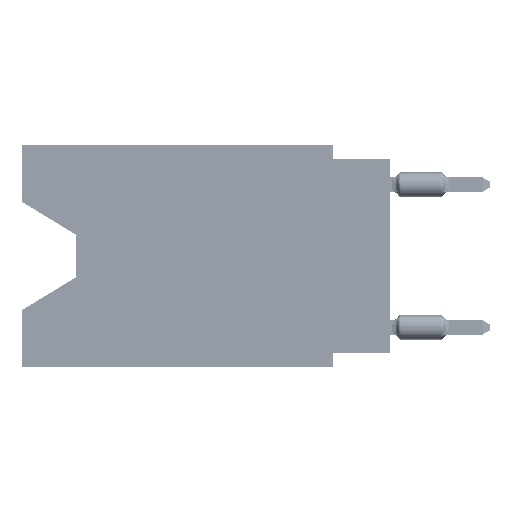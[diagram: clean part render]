
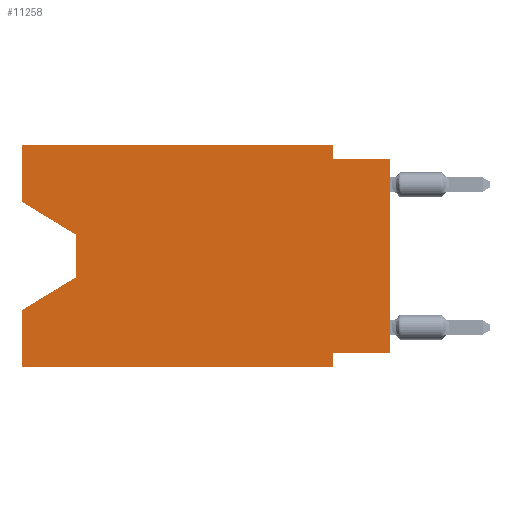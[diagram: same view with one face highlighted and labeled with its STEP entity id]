
A CAD part, left-side view. The second image highlights one B-rep face of the part: STEP entity #11258.
In plain terms, the highlighted planar face has unit normal (-1, 0, 0).
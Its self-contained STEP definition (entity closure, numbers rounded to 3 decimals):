
#1459 = EDGE_CURVE ( 'NONE', #8848, #53704, #19387, .T. ) ;
#1795 = CARTESIAN_POINT ( 'NONE',  ( 0., 2.54, 0. ) ) ;
#1817 = VECTOR ( 'NONE', #56384, 1000. ) ;
#1835 = VERTEX_POINT ( 'NONE', #5808 ) ;
#2385 = EDGE_CURVE ( 'NONE', #43833, #4414, #7277, .T. ) ;
#2601 = CARTESIAN_POINT ( 'NONE',  ( 0., 13.97, -5.893 ) ) ;
#3404 = FACE_OUTER_BOUND ( 'NONE', #23975, .T. ) ;
#3850 = LINE ( 'NONE', #23062, #57773 ) ;
#4297 = CARTESIAN_POINT ( 'NONE',  ( 0., 16.383, -9.906 ) ) ;
#4414 = VERTEX_POINT ( 'NONE', #1795 ) ;
#4616 = DIRECTION ( 'NONE',  ( 0., 1., 0. ) ) ;
#5125 = CARTESIAN_POINT ( 'NONE',  ( 0., 2.54, -9.906 ) ) ;
#5251 = DIRECTION ( 'NONE',  ( 0., -1., 0. ) ) ;
#5705 = CARTESIAN_POINT ( 'NONE',  ( 0., 16.383, -9.906 ) ) ;
#5808 = CARTESIAN_POINT ( 'NONE',  ( 0., 0., -0.635 ) ) ;
#5877 = CARTESIAN_POINT ( 'NONE',  ( 0., 16.383, 0. ) ) ;
#6912 = VERTEX_POINT ( 'NONE', #57296 ) ;
#7214 = DIRECTION ( 'NONE',  ( 0., 0., -1. ) ) ;
#7277 = LINE ( 'NONE', #31486, #11362 ) ;
#8170 = ORIENTED_EDGE ( 'NONE', *, *, #18318, .T. ) ;
#8647 = EDGE_CURVE ( 'NONE', #4414, #37309, #61099, .T. ) ;
#8848 = VERTEX_POINT ( 'NONE', #5705 ) ;
#9595 = ORIENTED_EDGE ( 'NONE', *, *, #14722, .F. ) ;
#11202 = VERTEX_POINT ( 'NONE', #56272 ) ;
#11258 = ADVANCED_FACE ( 'NONE', ( #3404 ), #16633, .F. ) ;
#11362 = VECTOR ( 'NONE', #49459, 1000. ) ;
#11464 = VECTOR ( 'NONE', #43907, 1000. ) ;
#12259 = CARTESIAN_POINT ( 'NONE',  ( 0., 0., -9.271 ) ) ;
#13710 = DIRECTION ( 'NONE',  ( 0., 0., 1. ) ) ;
#14200 = ORIENTED_EDGE ( 'NONE', *, *, #18834, .T. ) ;
#14722 = EDGE_CURVE ( 'NONE', #30793, #43833, #3850, .T. ) ;
#14852 = LINE ( 'NONE', #5125, #23028 ) ;
#14898 = ORIENTED_EDGE ( 'NONE', *, *, #27889, .T. ) ;
#15751 = CARTESIAN_POINT ( 'NONE',  ( 0., 16.383, 0. ) ) ;
#16633 = PLANE ( 'NONE',  #61138 ) ;
#18259 = VECTOR ( 'NONE', #29150, 1000. ) ;
#18318 = EDGE_CURVE ( 'NONE', #54765, #53704, #20858, .T. ) ;
#18834 = EDGE_CURVE ( 'NONE', #30793, #44508, #41213, .T. ) ;
#18895 = EDGE_CURVE ( 'NONE', #11202, #26272, #23185, .T. ) ;
#19387 = LINE ( 'NONE', #5877, #18259 ) ;
#19645 = ORIENTED_EDGE ( 'NONE', *, *, #20628, .T. ) ;
#19694 = VECTOR ( 'NONE', #59568, 1000. ) ;
#20628 = EDGE_CURVE ( 'NONE', #8848, #6912, #62211, .T. ) ;
#20858 = LINE ( 'NONE', #2601, #19694 ) ;
#22007 = ORIENTED_EDGE ( 'NONE', *, *, #57055, .F. ) ;
#22021 = DIRECTION ( 'NONE',  ( 0., -0.855, -0.519 ) ) ;
#23028 = VECTOR ( 'NONE', #48539, 1000. ) ;
#23062 = CARTESIAN_POINT ( 'NONE',  ( 0., 16.383, 0. ) ) ;
#23175 = LINE ( 'NONE', #27587, #49689 ) ;
#23185 = LINE ( 'NONE', #12259, #54922 ) ;
#23975 = EDGE_LOOP ( 'NONE', ( #14200, #14898, #8170, #43128, #19645, #51149, #30018, #38685, #22007, #46009, #32661, #9595 ) ) ;
#25698 = DIRECTION ( 'NONE',  ( 0., 0., 1. ) ) ;
#26272 = VERTEX_POINT ( 'NONE', #46825 ) ;
#27587 = CARTESIAN_POINT ( 'NONE',  ( 0., 0., 0. ) ) ;
#27889 = EDGE_CURVE ( 'NONE', #44508, #54765, #58396, .T. ) ;
#29150 = DIRECTION ( 'NONE',  ( 0., 0., 1. ) ) ;
#29646 = CARTESIAN_POINT ( 'NONE',  ( 0., 16.383, -2.546 ) ) ;
#30018 = ORIENTED_EDGE ( 'NONE', *, *, #18895, .F. ) ;
#30793 = VERTEX_POINT ( 'NONE', #29646 ) ;
#31441 = CARTESIAN_POINT ( 'NONE',  ( 0., 13.97, -5.893 ) ) ;
#31486 = CARTESIAN_POINT ( 'NONE',  ( 0., 16.383, 0. ) ) ;
#32661 = ORIENTED_EDGE ( 'NONE', *, *, #2385, .F. ) ;
#34424 = EDGE_CURVE ( 'NONE', #26272, #6912, #14852, .T. ) ;
#34960 = CARTESIAN_POINT ( 'NONE',  ( 0., 2.54, -0.635 ) ) ;
#34983 = VECTOR ( 'NONE', #5251, 1000. ) ;
#36754 = CARTESIAN_POINT ( 'NONE',  ( 0., 0., -0.635 ) ) ;
#37309 = VERTEX_POINT ( 'NONE', #34960 ) ;
#37951 = CARTESIAN_POINT ( 'NONE',  ( 0., 16.383, -2.546 ) ) ;
#38685 = ORIENTED_EDGE ( 'NONE', *, *, #56535, .T. ) ;
#39481 = CARTESIAN_POINT ( 'NONE',  ( 0., 13.97, -4.013 ) ) ;
#41160 = LINE ( 'NONE', #36754, #50753 ) ;
#41213 = LINE ( 'NONE', #37951, #58976 ) ;
#41781 = DIRECTION ( 'NONE',  ( 0., -1., 0. ) ) ;
#43128 = ORIENTED_EDGE ( 'NONE', *, *, #1459, .F. ) ;
#43833 = VERTEX_POINT ( 'NONE', #15751 ) ;
#43907 = DIRECTION ( 'NONE',  ( 0., 0., -1. ) ) ;
#44508 = VERTEX_POINT ( 'NONE', #39481 ) ;
#46009 = ORIENTED_EDGE ( 'NONE', *, *, #8647, .F. ) ;
#46328 = CARTESIAN_POINT ( 'NONE',  ( 0., 2.54, 0. ) ) ;
#46825 = CARTESIAN_POINT ( 'NONE',  ( 0., 2.54, -9.271 ) ) ;
#48539 = DIRECTION ( 'NONE',  ( 0., 0., -1. ) ) ;
#49459 = DIRECTION ( 'NONE',  ( 0., -1., 0. ) ) ;
#49689 = VECTOR ( 'NONE', #13710, 1000. ) ;
#50307 = DIRECTION ( 'NONE',  ( 1., 0., 0. ) ) ;
#50612 = CARTESIAN_POINT ( 'NONE',  ( 0., 16.383, 0. ) ) ;
#50753 = VECTOR ( 'NONE', #41781, 1000. ) ;
#51149 = ORIENTED_EDGE ( 'NONE', *, *, #34424, .F. ) ;
#53704 = VERTEX_POINT ( 'NONE', #58390 ) ;
#54765 = VERTEX_POINT ( 'NONE', #31441 ) ;
#54922 = VECTOR ( 'NONE', #4616, 1000. ) ;
#56272 = CARTESIAN_POINT ( 'NONE',  ( 0., 0., -9.271 ) ) ;
#56384 = DIRECTION ( 'NONE',  ( 0., 0., -1. ) ) ;
#56535 = EDGE_CURVE ( 'NONE', #11202, #1835, #23175, .T. ) ;
#57055 = EDGE_CURVE ( 'NONE', #37309, #1835, #41160, .T. ) ;
#57296 = CARTESIAN_POINT ( 'NONE',  ( 0., 2.54, -9.906 ) ) ;
#57773 = VECTOR ( 'NONE', #25698, 1000. ) ;
#58390 = CARTESIAN_POINT ( 'NONE',  ( 0., 16.383, -7.36 ) ) ;
#58396 = LINE ( 'NONE', #58712, #11464 ) ;
#58712 = CARTESIAN_POINT ( 'NONE',  ( 0., 13.97, -4.013 ) ) ;
#58976 = VECTOR ( 'NONE', #22021, 1000. ) ;
#59568 = DIRECTION ( 'NONE',  ( 0., 0.855, -0.519 ) ) ;
#61099 = LINE ( 'NONE', #46328, #1817 ) ;
#61138 = AXIS2_PLACEMENT_3D ( 'NONE', #50612, #50307, #7214 ) ;
#62211 = LINE ( 'NONE', #4297, #34983 ) ;
